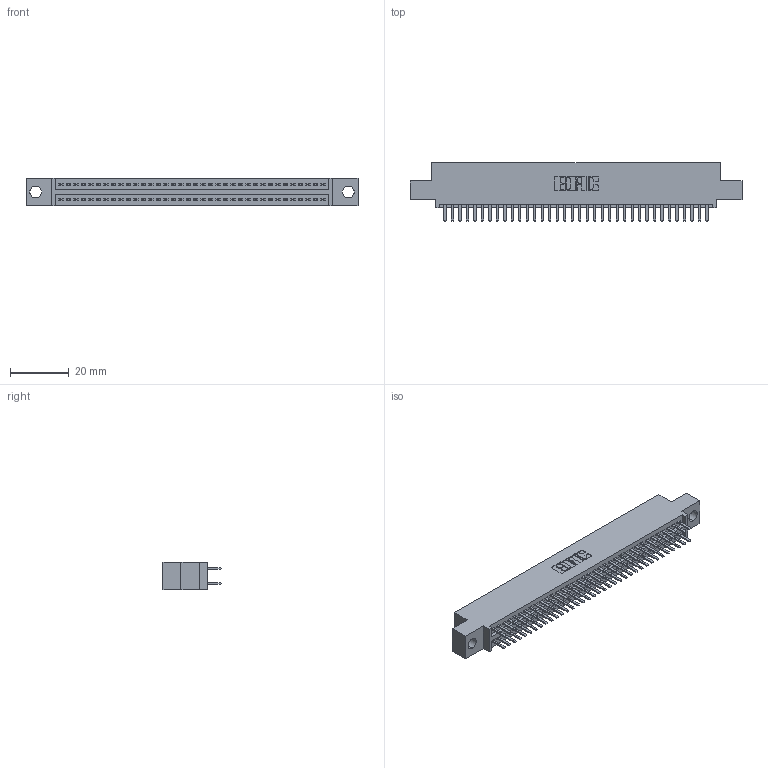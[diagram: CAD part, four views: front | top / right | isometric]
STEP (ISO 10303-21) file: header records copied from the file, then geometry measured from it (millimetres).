
FILE_DESCRIPTION (( 'STEP AP203' ), '1' );
FILE_NAME ('345-072-520-504.STEP', '2018-10-02T03:32:10', ( '' ), ( '' ), 'SwSTEP 2.0', 'SolidWorks 2016', '' );
FILE_SCHEMA (( 'CONFIG_CONTROL_DESIGN' ));
Length unit declared in the file: inch
Products named in the file (3): 345-292-001_345-293-120; 345 Part_0.110 Offset - 0.156 Dia-TH; 345-072-520-504
Assembly tree (73 placements, depth 2):
  345-072-520-504
    345 Part_0.110 Offset - 0.156 Dia-TH
    345-292-001_345-293-120  x72
Bounding box: 112.65 x 19.68 x 9.4 mm (x, y, z)
Volume: 10694.3 mm3; surface area: 15532.4 mm2
Topology: 73 solids, 73 shells, 4018 faces, 11657 edges, 7578 vertices
Faces by surface type: plane 2604, cylinder 1414
Entity records: 29303 total; most frequent: CARTESIAN_POINT 4932, ORIENTED_EDGE 4854, DIRECTION 4343, EDGE_CURVE 2427, LINE 2147, VECTOR 2147, VERTEX_POINT 1614, AXIS2_PLACEMENT_3D 1098
